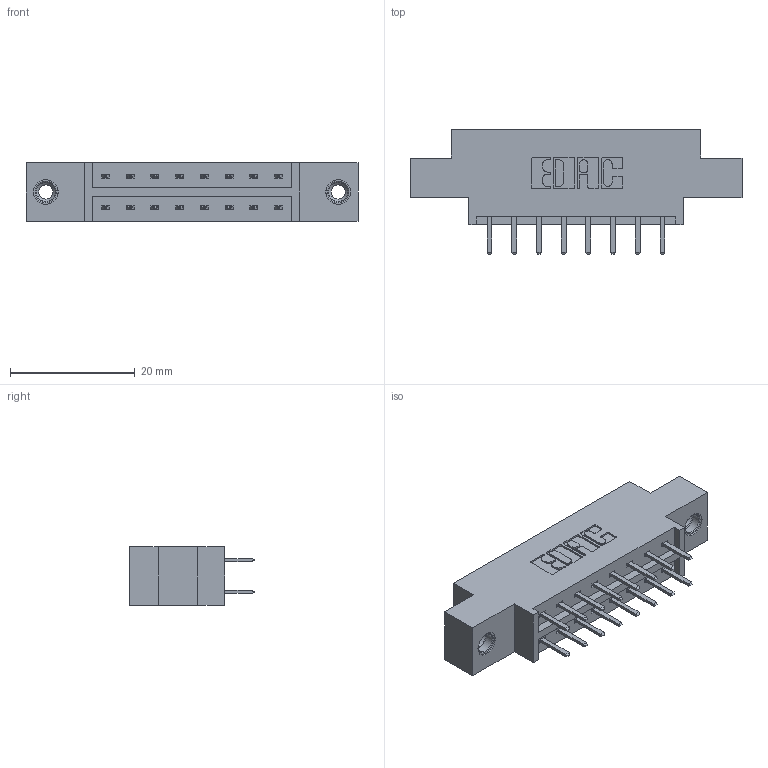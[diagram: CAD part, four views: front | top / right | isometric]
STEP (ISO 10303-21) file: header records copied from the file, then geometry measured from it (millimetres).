
FILE_DESCRIPTION (( 'STEP AP203' ), '1' );
FILE_NAME ('833-016-520-808.STEP', '2020-05-31T16:59:28', ( '' ), ( '' ), 'SwSTEP 2.0', 'SolidWorks 2020', '' );
FILE_SCHEMA (( 'CONFIG_CONTROL_DESIGN' ));
Length unit declared in the file: inch
Products named in the file (4): 345-292-001_345-293-120; 833-016-520-808; 833 Part_Offset - .156 Dia - TI; 345-250-001_345-250-003-102
Assembly tree (19 placements, depth 2):
  833-016-520-808
    833 Part_Offset - .156 Dia - TI
    345-292-001_345-293-120  x16
    345-250-001_345-250-003-102  x2
Bounding box: 53.24 x 20.02 x 9.4 mm (x, y, z)
Volume: 4876 mm3; surface area: 5623.3 mm2
Topology: 19 solids, 19 shells, 1074 faces, 3067 edges, 1994 vertices
Faces by surface type: plane 714, cylinder 344, cone 12, torus 4
Entity records: 10976 total; most frequent: CARTESIAN_POINT 1857, ORIENTED_EDGE 1774, DIRECTION 1665, EDGE_CURVE 887, LINE 735, VECTOR 735, VERTEX_POINT 584, AXIS2_PLACEMENT_3D 465
